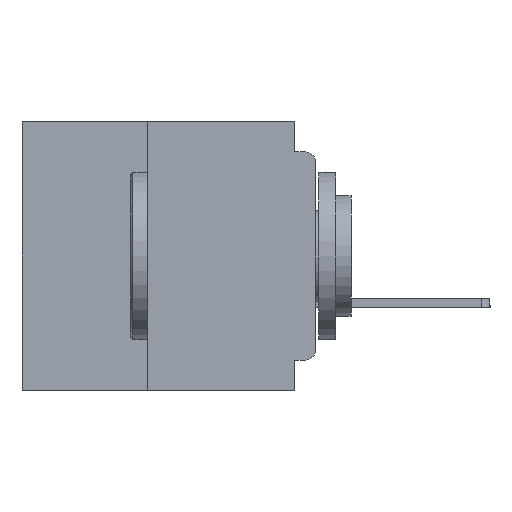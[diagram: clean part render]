
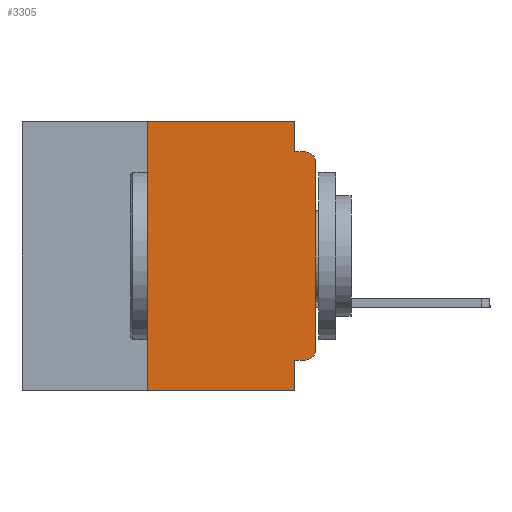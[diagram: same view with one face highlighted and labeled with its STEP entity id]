
A CAD part, left-side view. The second image highlights one B-rep face of the part: STEP entity #3305.
In plain terms, the highlighted planar face has unit normal (-1, 0, 0).
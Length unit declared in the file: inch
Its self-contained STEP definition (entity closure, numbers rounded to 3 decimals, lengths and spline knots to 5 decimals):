
#130 = CIRCLE ( 'NONE', #46960, 0.015 ) ;
#2555 = DIRECTION ( 'NONE',  ( 0., 1., 0. ) ) ;
#2836 = CARTESIAN_POINT ( 'NONE',  ( 0., 0.437, -0.4 ) ) ;
#2852 = ORIENTED_EDGE ( 'NONE', *, *, #55702, .F. ) ;
#2880 = EDGE_CURVE ( 'NONE', #49044, #31395, #23831, .T. ) ;
#2919 = VERTEX_POINT ( 'NONE', #32263 ) ;
#2920 = DIRECTION ( 'NONE',  ( 0., 0., 1. ) ) ;
#3305 = ADVANCED_FACE ( 'NONE', ( #34892 ), #58448, .F. ) ;
#3437 = VERTEX_POINT ( 'NONE', #36364 ) ;
#4329 = LINE ( 'NONE', #7215, #15445 ) ;
#5185 = CARTESIAN_POINT ( 'NONE',  ( 0., 0.015, -0.34 ) ) ;
#5198 = VECTOR ( 'NONE', #45306, 39.37008 ) ;
#5652 = VERTEX_POINT ( 'NONE', #37983 ) ;
#7215 = CARTESIAN_POINT ( 'NONE',  ( 0., 0., -0.045 ) ) ;
#7240 = EDGE_CURVE ( 'NONE', #38636, #5652, #51026, .T. ) ;
#7733 = CARTESIAN_POINT ( 'NONE',  ( 0., 0.25, -0.4 ) ) ;
#9930 = DIRECTION ( 'NONE',  ( 0., 0., -1. ) ) ;
#10371 = CARTESIAN_POINT ( 'NONE',  ( 0., 0., -0.06 ) ) ;
#10858 = EDGE_CURVE ( 'NONE', #47097, #49044, #60832, .T. ) ;
#11053 = EDGE_CURVE ( 'NONE', #2919, #35168, #58604, .T. ) ;
#11416 = CARTESIAN_POINT ( 'NONE',  ( 0., 0.437, 0. ) ) ;
#11995 = DIRECTION ( 'NONE',  ( 0., -1., 0. ) ) ;
#12242 = CARTESIAN_POINT ( 'NONE',  ( 0., 0.25, -0.4 ) ) ;
#12291 = VERTEX_POINT ( 'NONE', #46650 ) ;
#12425 = DIRECTION ( 'NONE',  ( 0., 0., 1. ) ) ;
#13115 = DIRECTION ( 'NONE',  ( -1., 0., 0. ) ) ;
#15445 = VECTOR ( 'NONE', #11995, 39.37008 ) ;
#16162 = DIRECTION ( 'NONE',  ( 1., 0., 0. ) ) ;
#17103 = AXIS2_PLACEMENT_3D ( 'NONE', #41359, #13115, #46064 ) ;
#18888 = EDGE_CURVE ( 'NONE', #3437, #58997, #55527, .T. ) ;
#20716 = LINE ( 'NONE', #2836, #5198 ) ;
#22282 = ORIENTED_EDGE ( 'NONE', *, *, #26271, .F. ) ;
#23831 = CIRCLE ( 'NONE', #17103, 0.015 ) ;
#24593 = DIRECTION ( 'NONE',  ( 0., 0., -1. ) ) ;
#25830 = CARTESIAN_POINT ( 'NONE',  ( 0., 0., -0.355 ) ) ;
#26271 = EDGE_CURVE ( 'NONE', #5652, #2919, #53899, .T. ) ;
#26720 = EDGE_CURVE ( 'NONE', #38636, #12291, #20716, .T. ) ;
#28056 = ORIENTED_EDGE ( 'NONE', *, *, #39219, .F. ) ;
#28698 = EDGE_LOOP ( 'NONE', ( #29080, #58798, #28056, #30455, #22282, #42125, #37319, #2852, #43930, #48289 ) ) ;
#29037 = VECTOR ( 'NONE', #2555, 39.37008 ) ;
#29080 = ORIENTED_EDGE ( 'NONE', *, *, #10858, .T. ) ;
#30368 = DIRECTION ( 'NONE',  ( 0., 0., -1. ) ) ;
#30455 = ORIENTED_EDGE ( 'NONE', *, *, #11053, .F. ) ;
#30911 = EDGE_CURVE ( 'NONE', #3437, #47097, #130, .T. ) ;
#31161 = CARTESIAN_POINT ( 'NONE',  ( 0., 0., 0. ) ) ;
#31395 = VERTEX_POINT ( 'NONE', #60242 ) ;
#32263 = CARTESIAN_POINT ( 'NONE',  ( 0., 0.031, 0. ) ) ;
#32344 = VECTOR ( 'NONE', #24593, 39.37008 ) ;
#32797 = DIRECTION ( 'NONE',  ( 0., 0., -1. ) ) ;
#34563 = CARTESIAN_POINT ( 'NONE',  ( 0., 0.031, -0.045 ) ) ;
#34892 = FACE_OUTER_BOUND ( 'NONE', #28698, .T. ) ;
#35168 = VERTEX_POINT ( 'NONE', #34563 ) ;
#36364 = CARTESIAN_POINT ( 'NONE',  ( 0., 0.015, -0.355 ) ) ;
#37319 = ORIENTED_EDGE ( 'NONE', *, *, #26720, .T. ) ;
#37983 = CARTESIAN_POINT ( 'NONE',  ( 0., 0.25, 0. ) ) ;
#38211 = DIRECTION ( 'NONE',  ( -1., 0., 0. ) ) ;
#38547 = VECTOR ( 'NONE', #2920, 39.37008 ) ;
#38636 = VERTEX_POINT ( 'NONE', #7733 ) ;
#39219 = EDGE_CURVE ( 'NONE', #35168, #31395, #4329, .T. ) ;
#41359 = CARTESIAN_POINT ( 'NONE',  ( 0., 0.015, -0.06 ) ) ;
#41454 = VECTOR ( 'NONE', #51503, 39.37008 ) ;
#42125 = ORIENTED_EDGE ( 'NONE', *, *, #7240, .F. ) ;
#43930 = ORIENTED_EDGE ( 'NONE', *, *, #18888, .F. ) ;
#44362 = AXIS2_PLACEMENT_3D ( 'NONE', #11416, #16162, #30368 ) ;
#44882 = LINE ( 'NONE', #57471, #32344 ) ;
#45306 = DIRECTION ( 'NONE',  ( 0., -1., 0. ) ) ;
#46064 = DIRECTION ( 'NONE',  ( 0., 0., -1. ) ) ;
#46202 = VECTOR ( 'NONE', #32797, 39.37008 ) ;
#46210 = CARTESIAN_POINT ( 'NONE',  ( 0., 0., -0.34 ) ) ;
#46650 = CARTESIAN_POINT ( 'NONE',  ( 0., 0.031, -0.4 ) ) ;
#46796 = CARTESIAN_POINT ( 'NONE',  ( 0., 0.437, 0. ) ) ;
#46960 = AXIS2_PLACEMENT_3D ( 'NONE', #5185, #38211, #9930 ) ;
#47097 = VERTEX_POINT ( 'NONE', #46210 ) ;
#48289 = ORIENTED_EDGE ( 'NONE', *, *, #30911, .T. ) ;
#49044 = VERTEX_POINT ( 'NONE', #10371 ) ;
#51026 = LINE ( 'NONE', #12242, #38547 ) ;
#51502 = CARTESIAN_POINT ( 'NONE',  ( 0., 0.031, 0. ) ) ;
#51503 = DIRECTION ( 'NONE',  ( 0., -1., 0. ) ) ;
#53899 = LINE ( 'NONE', #46796, #41454 ) ;
#55527 = LINE ( 'NONE', #25830, #29037 ) ;
#55702 = EDGE_CURVE ( 'NONE', #58997, #12291, #44882, .T. ) ;
#56017 = CARTESIAN_POINT ( 'NONE',  ( 0., 0.031, -0.355 ) ) ;
#57471 = CARTESIAN_POINT ( 'NONE',  ( 0., 0.031, -0.4 ) ) ;
#57903 = VECTOR ( 'NONE', #12425, 39.37008 ) ;
#58448 = PLANE ( 'NONE',  #44362 ) ;
#58604 = LINE ( 'NONE', #51502, #46202 ) ;
#58798 = ORIENTED_EDGE ( 'NONE', *, *, #2880, .T. ) ;
#58997 = VERTEX_POINT ( 'NONE', #56017 ) ;
#60242 = CARTESIAN_POINT ( 'NONE',  ( 0., 0.015, -0.045 ) ) ;
#60832 = LINE ( 'NONE', #31161, #57903 ) ;
